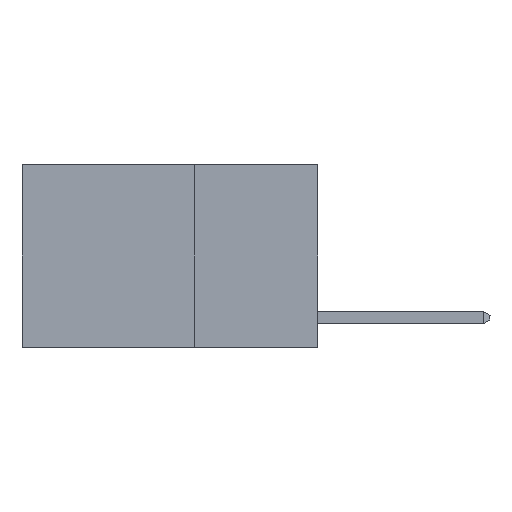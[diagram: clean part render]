
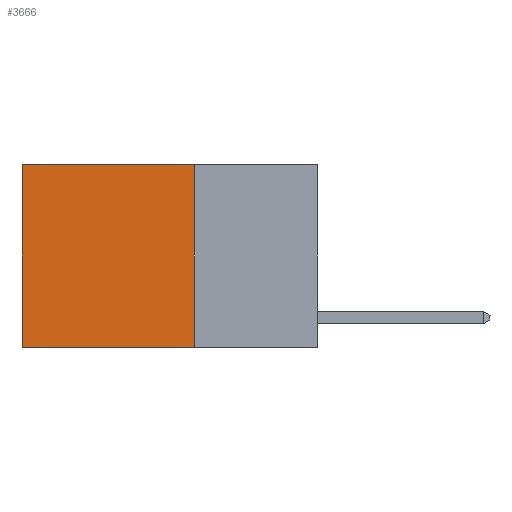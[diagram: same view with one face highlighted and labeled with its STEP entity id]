
A CAD part, left-side view. The second image highlights one B-rep face of the part: STEP entity #3666.
In plain terms, the highlighted planar face has unit normal (-1, 0, 0).
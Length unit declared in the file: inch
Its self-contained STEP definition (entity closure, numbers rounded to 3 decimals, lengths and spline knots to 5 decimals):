
#190 = CARTESIAN_POINT ( 'NONE',  ( 0.2625, 0.25, 0. ) ) ;
#1439 = CARTESIAN_POINT ( 'NONE',  ( 0.2625, 0.6, -0.37 ) ) ;
#2019 = DIRECTION ( 'NONE',  ( 0., 1., 0. ) ) ;
#2132 = LINE ( 'NONE', #190, #19743 ) ;
#2309 = CARTESIAN_POINT ( 'NONE',  ( 0.2625, 0.6, 0. ) ) ;
#3666 = ADVANCED_FACE ( 'NONE', ( #7597 ), #26782, .F. ) ;
#7597 = FACE_OUTER_BOUND ( 'NONE', #16225, .T. ) ;
#7995 = DIRECTION ( 'NONE',  ( 1., 0., 0. ) ) ;
#8076 = ORIENTED_EDGE ( 'NONE', *, *, #21028, .F. ) ;
#8947 = VERTEX_POINT ( 'NONE', #23024 ) ;
#10624 = VECTOR ( 'NONE', #2019, 39.37008 ) ;
#11788 = CARTESIAN_POINT ( 'NONE',  ( 0.2625, 0.25, 0. ) ) ;
#12355 = LINE ( 'NONE', #2309, #18863 ) ;
#13133 = VERTEX_POINT ( 'NONE', #22878 ) ;
#15842 = EDGE_CURVE ( 'NONE', #8947, #22215, #27199, .T. ) ;
#16107 = VERTEX_POINT ( 'NONE', #1439 ) ;
#16225 = EDGE_LOOP ( 'NONE', ( #23456, #22727, #8076, #17527 ) ) ;
#17155 = EDGE_CURVE ( 'NONE', #13133, #16107, #18244, .T. ) ;
#17527 = ORIENTED_EDGE ( 'NONE', *, *, #15842, .T. ) ;
#18118 = CARTESIAN_POINT ( 'NONE',  ( 0.2625, 0.25, -0.37 ) ) ;
#18244 = LINE ( 'NONE', #18118, #19151 ) ;
#18466 = DIRECTION ( 'NONE',  ( 0., 0., -1. ) ) ;
#18863 = VECTOR ( 'NONE', #25289, 39.37008 ) ;
#19151 = VECTOR ( 'NONE', #20198, 39.37008 ) ;
#19743 = VECTOR ( 'NONE', #20964, 39.37008 ) ;
#20198 = DIRECTION ( 'NONE',  ( 0., 1., 0. ) ) ;
#20964 = DIRECTION ( 'NONE',  ( 0., 0., -1. ) ) ;
#21028 = EDGE_CURVE ( 'NONE', #8947, #13133, #2132, .T. ) ;
#21154 = CARTESIAN_POINT ( 'NONE',  ( 0.2625, 0.25, 0. ) ) ;
#21618 = EDGE_CURVE ( 'NONE', #22215, #16107, #12355, .T. ) ;
#22215 = VERTEX_POINT ( 'NONE', #23977 ) ;
#22727 = ORIENTED_EDGE ( 'NONE', *, *, #17155, .F. ) ;
#22878 = CARTESIAN_POINT ( 'NONE',  ( 0.2625, 0.25, -0.37 ) ) ;
#23024 = CARTESIAN_POINT ( 'NONE',  ( 0.2625, 0.25, 0. ) ) ;
#23456 = ORIENTED_EDGE ( 'NONE', *, *, #21618, .T. ) ;
#23977 = CARTESIAN_POINT ( 'NONE',  ( 0.2625, 0.6, 0. ) ) ;
#24186 = AXIS2_PLACEMENT_3D ( 'NONE', #11788, #7995, #18466 ) ;
#25289 = DIRECTION ( 'NONE',  ( 0., 0., -1. ) ) ;
#26782 = PLANE ( 'NONE',  #24186 ) ;
#27199 = LINE ( 'NONE', #21154, #10624 ) ;
